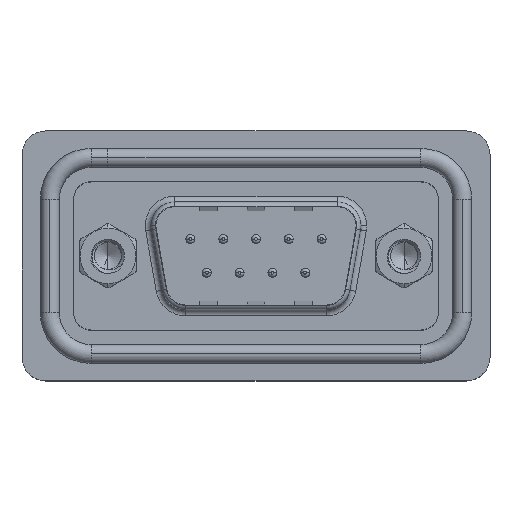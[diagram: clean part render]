
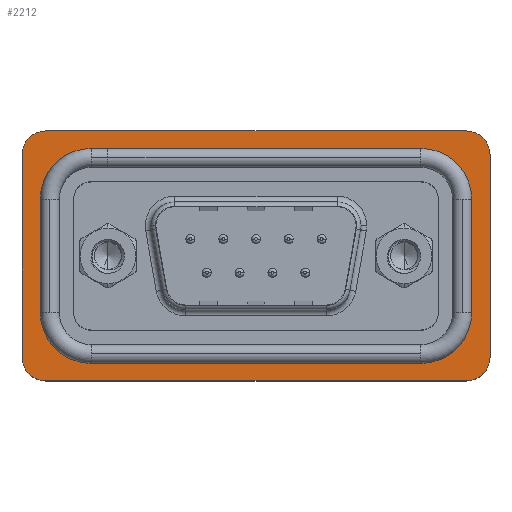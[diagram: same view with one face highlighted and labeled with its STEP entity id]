
A CAD part, top view. The second image highlights one B-rep face of the part: STEP entity #2212.
In plain terms, the highlighted planar face has unit normal (0, 0, 1).
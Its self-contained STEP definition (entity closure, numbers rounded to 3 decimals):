
#7 = DIRECTION ( 'NONE',  ( 1., 0., 0. ) ) ;
#293 = VERTEX_POINT ( 'NONE', #15740 ) ;
#303 = DIRECTION ( 'NONE',  ( 0., -1., 0. ) ) ;
#667 = LINE ( 'NONE', #5369, #3096 ) ;
#698 = CARTESIAN_POINT ( 'NONE',  ( 26.405, 9.075, 0.5 ) ) ;
#702 = CARTESIAN_POINT ( 'NONE',  ( -5.25, 10.55, 0.5 ) ) ;
#779 = VERTEX_POINT ( 'NONE', #1480 ) ;
#960 = CARTESIAN_POINT ( 'NONE',  ( -5.25, -8.55, 0.5 ) ) ;
#1004 = CARTESIAN_POINT ( 'NONE',  ( 26.405, -9.075, 0.5 ) ) ;
#1094 = VECTOR ( 'NONE', #3246, 1000. ) ;
#1358 = ORIENTED_EDGE ( 'NONE', *, *, #5745, .F. ) ;
#1480 = CARTESIAN_POINT ( 'NONE',  ( 30.705, -4.775, 0.5 ) ) ;
#1558 = CIRCLE ( 'NONE', #3838, 2. ) ;
#1612 = ORIENTED_EDGE ( 'NONE', *, *, #15712, .F. ) ;
#1641 = CARTESIAN_POINT ( 'NONE',  ( -1.405, 9.075, 0.5 ) ) ;
#1839 = LINE ( 'NONE', #8086, #11304 ) ;
#2130 = LINE ( 'NONE', #15849, #5525 ) ;
#2212 = ADVANCED_FACE ( 'NONE', ( #6549, #6759 ), #11276, .T. ) ;
#2410 = AXIS2_PLACEMENT_3D ( 'NONE', #3085, #6654, #7 ) ;
#2508 = VERTEX_POINT ( 'NONE', #20027 ) ;
#2511 = DIRECTION ( 'NONE',  ( -1., 0., 0. ) ) ;
#2998 = EDGE_CURVE ( 'NONE', #5143, #14491, #10978, .T. ) ;
#3085 = CARTESIAN_POINT ( 'NONE',  ( -1.405, -4.775, 0.5 ) ) ;
#3096 = VECTOR ( 'NONE', #2511, 1000. ) ;
#3149 = LINE ( 'NONE', #4671, #8349 ) ;
#3159 = ORIENTED_EDGE ( 'NONE', *, *, #10698, .T. ) ;
#3246 = DIRECTION ( 'NONE',  ( 0., 1., 0. ) ) ;
#3379 = DIRECTION ( 'NONE',  ( 1., 0., 0. ) ) ;
#3398 = VECTOR ( 'NONE', #16987, 1000. ) ;
#3555 = DIRECTION ( 'NONE',  ( 1., 0., 0. ) ) ;
#3666 = DIRECTION ( 'NONE',  ( 0., 0., 1. ) ) ;
#3838 = AXIS2_PLACEMENT_3D ( 'NONE', #17685, #3666, #9921 ) ;
#3862 = EDGE_CURVE ( 'NONE', #11667, #16319, #6385, .T. ) ;
#3866 = CIRCLE ( 'NONE', #14004, 2. ) ;
#3892 = CARTESIAN_POINT ( 'NONE',  ( 32.25, -8.55, 0.5 ) ) ;
#4145 = ORIENTED_EDGE ( 'NONE', *, *, #11080, .F. ) ;
#4476 = CIRCLE ( 'NONE', #15607, 2. ) ;
#4671 = CARTESIAN_POINT ( 'NONE',  ( 30.25, -10.55, 0.5 ) ) ;
#4672 = CARTESIAN_POINT ( 'NONE',  ( -1.405, 4.775, 0.5 ) ) ;
#5143 = VERTEX_POINT ( 'NONE', #17785 ) ;
#5189 = DIRECTION ( 'NONE',  ( 0., 0., 1. ) ) ;
#5277 = DIRECTION ( 'NONE',  ( 0., -1., 0. ) ) ;
#5358 = ORIENTED_EDGE ( 'NONE', *, *, #17830, .F. ) ;
#5361 = VERTEX_POINT ( 'NONE', #13994 ) ;
#5369 = CARTESIAN_POINT ( 'NONE',  ( 30.25, 10.55, 0.5 ) ) ;
#5525 = VECTOR ( 'NONE', #12693, 1000. ) ;
#5574 = EDGE_CURVE ( 'NONE', #16319, #2508, #9483, .T. ) ;
#5633 = VECTOR ( 'NONE', #5277, 1000. ) ;
#5745 = EDGE_CURVE ( 'NONE', #293, #19605, #14707, .T. ) ;
#5815 = VERTEX_POINT ( 'NONE', #11754 ) ;
#6047 = AXIS2_PLACEMENT_3D ( 'NONE', #16203, #12932, #17631 ) ;
#6385 = CIRCLE ( 'NONE', #17832, 2. ) ;
#6549 = FACE_BOUND ( 'NONE', #17944, .T. ) ;
#6555 = EDGE_CURVE ( 'NONE', #19605, #9737, #18405, .T. ) ;
#6643 = CARTESIAN_POINT ( 'NONE',  ( 30.25, 8.55, 0.5 ) ) ;
#6654 = DIRECTION ( 'NONE',  ( 0., 0., 1. ) ) ;
#6759 = FACE_OUTER_BOUND ( 'NONE', #15097, .T. ) ;
#6971 = CARTESIAN_POINT ( 'NONE',  ( 30.705, -4.775, 0.5 ) ) ;
#7002 = AXIS2_PLACEMENT_3D ( 'NONE', #6643, #9744, #3379 ) ;
#7195 = DIRECTION ( 'NONE',  ( 0., 0., 1. ) ) ;
#7319 = EDGE_CURVE ( 'NONE', #15814, #10655, #667, .T. ) ;
#7572 = LINE ( 'NONE', #15462, #3398 ) ;
#8086 = CARTESIAN_POINT ( 'NONE',  ( -7.25, -8.55, 0.5 ) ) ;
#8247 = CARTESIAN_POINT ( 'NONE',  ( 32.25, -8.55, 0.5 ) ) ;
#8293 = CARTESIAN_POINT ( 'NONE',  ( 30.25, -8.55, 0.5 ) ) ;
#8349 = VECTOR ( 'NONE', #12568, 1000. ) ;
#8527 = ORIENTED_EDGE ( 'NONE', *, *, #17581, .T. ) ;
#8582 = EDGE_CURVE ( 'NONE', #10655, #5815, #4476, .T. ) ;
#8651 = CARTESIAN_POINT ( 'NONE',  ( -5.705, 4.775, 0.5 ) ) ;
#8803 = CARTESIAN_POINT ( 'NONE',  ( -5.25, 8.55, 0.5 ) ) ;
#9399 = CIRCLE ( 'NONE', #13975, 4.3 ) ;
#9483 = LINE ( 'NONE', #8247, #1094 ) ;
#9565 = ORIENTED_EDGE ( 'NONE', *, *, #5574, .T. ) ;
#9657 = AXIS2_PLACEMENT_3D ( 'NONE', #15427, #15731, #20118 ) ;
#9737 = VERTEX_POINT ( 'NONE', #15664 ) ;
#9744 = DIRECTION ( 'NONE',  ( 0., 0., 1. ) ) ;
#9921 = DIRECTION ( 'NONE',  ( 1., 0., 0. ) ) ;
#10398 = ORIENTED_EDGE ( 'NONE', *, *, #2998, .F. ) ;
#10655 = VERTEX_POINT ( 'NONE', #702 ) ;
#10698 = EDGE_CURVE ( 'NONE', #2508, #15814, #1558, .T. ) ;
#10743 = DIRECTION ( 'NONE',  ( 0., 0., 1. ) ) ;
#10783 = VERTEX_POINT ( 'NONE', #1004 ) ;
#10978 = CIRCLE ( 'NONE', #6047, 4.3 ) ;
#11014 = CARTESIAN_POINT ( 'NONE',  ( -5.705, -4.775, 0.5 ) ) ;
#11080 = EDGE_CURVE ( 'NONE', #11955, #293, #9399, .T. ) ;
#11276 = PLANE ( 'NONE',  #7002 ) ;
#11304 = VECTOR ( 'NONE', #303, 1000. ) ;
#11609 = LINE ( 'NONE', #6971, #14509 ) ;
#11667 = VERTEX_POINT ( 'NONE', #12847 ) ;
#11754 = CARTESIAN_POINT ( 'NONE',  ( -7.25, 8.55, 0.5 ) ) ;
#11765 = EDGE_CURVE ( 'NONE', #17710, #5361, #3866, .T. ) ;
#11808 = ORIENTED_EDGE ( 'NONE', *, *, #11765, .T. ) ;
#11955 = VERTEX_POINT ( 'NONE', #1641 ) ;
#12568 = DIRECTION ( 'NONE',  ( 1., 0., 0. ) ) ;
#12669 = EDGE_CURVE ( 'NONE', #9737, #10783, #2130, .T. ) ;
#12693 = DIRECTION ( 'NONE',  ( 1., 0., 0. ) ) ;
#12847 = CARTESIAN_POINT ( 'NONE',  ( 30.25, -10.55, 0.5 ) ) ;
#12932 = DIRECTION ( 'NONE',  ( 0., 0., 1. ) ) ;
#13081 = ORIENTED_EDGE ( 'NONE', *, *, #7319, .T. ) ;
#13525 = DIRECTION ( 'NONE',  ( 0., 1., 0. ) ) ;
#13901 = CIRCLE ( 'NONE', #9657, 4.3 ) ;
#13975 = AXIS2_PLACEMENT_3D ( 'NONE', #4672, #5189, #3555 ) ;
#13994 = CARTESIAN_POINT ( 'NONE',  ( -5.25, -10.55, 0.5 ) ) ;
#14004 = AXIS2_PLACEMENT_3D ( 'NONE', #960, #7195, #16983 ) ;
#14094 = CARTESIAN_POINT ( 'NONE',  ( -7.25, -8.55, 0.5 ) ) ;
#14473 = ORIENTED_EDGE ( 'NONE', *, *, #12669, .F. ) ;
#14491 = VERTEX_POINT ( 'NONE', #698 ) ;
#14509 = VECTOR ( 'NONE', #13525, 1000. ) ;
#14707 = LINE ( 'NONE', #8651, #5633 ) ;
#14765 = CARTESIAN_POINT ( 'NONE',  ( 30.25, 10.55, 0.5 ) ) ;
#15097 = EDGE_LOOP ( 'NONE', ( #3159, #13081, #20128, #8527, #11808, #18176, #20076, #9565 ) ) ;
#15152 = ORIENTED_EDGE ( 'NONE', *, *, #6555, .F. ) ;
#15427 = CARTESIAN_POINT ( 'NONE',  ( 26.405, -4.775, 0.5 ) ) ;
#15462 = CARTESIAN_POINT ( 'NONE',  ( 26.405, 9.075, 0.5 ) ) ;
#15607 = AXIS2_PLACEMENT_3D ( 'NONE', #8803, #10743, #16972 ) ;
#15664 = CARTESIAN_POINT ( 'NONE',  ( -1.405, -9.075, 0.5 ) ) ;
#15712 = EDGE_CURVE ( 'NONE', #779, #5143, #11609, .T. ) ;
#15731 = DIRECTION ( 'NONE',  ( 0., 0., 1. ) ) ;
#15740 = CARTESIAN_POINT ( 'NONE',  ( -5.705, 4.775, 0.5 ) ) ;
#15814 = VERTEX_POINT ( 'NONE', #14765 ) ;
#15836 = EDGE_CURVE ( 'NONE', #14491, #11955, #7572, .T. ) ;
#15849 = CARTESIAN_POINT ( 'NONE',  ( -1.405, -9.075, 0.5 ) ) ;
#15873 = DIRECTION ( 'NONE',  ( 0., 0., 1. ) ) ;
#16203 = CARTESIAN_POINT ( 'NONE',  ( 26.405, 4.775, 0.5 ) ) ;
#16319 = VERTEX_POINT ( 'NONE', #3892 ) ;
#16972 = DIRECTION ( 'NONE',  ( 1., 0., 0. ) ) ;
#16983 = DIRECTION ( 'NONE',  ( -1., 0., 0. ) ) ;
#16987 = DIRECTION ( 'NONE',  ( -1., 0., 0. ) ) ;
#17581 = EDGE_CURVE ( 'NONE', #5815, #17710, #1839, .T. ) ;
#17631 = DIRECTION ( 'NONE',  ( 1., 0., 0. ) ) ;
#17685 = CARTESIAN_POINT ( 'NONE',  ( 30.25, 8.55, 0.5 ) ) ;
#17710 = VERTEX_POINT ( 'NONE', #14094 ) ;
#17785 = CARTESIAN_POINT ( 'NONE',  ( 30.705, 4.775, 0.5 ) ) ;
#17830 = EDGE_CURVE ( 'NONE', #10783, #779, #13901, .T. ) ;
#17832 = AXIS2_PLACEMENT_3D ( 'NONE', #8293, #15873, #19038 ) ;
#17944 = EDGE_LOOP ( 'NONE', ( #10398, #1612, #5358, #14473, #15152, #1358, #4145, #18035 ) ) ;
#18035 = ORIENTED_EDGE ( 'NONE', *, *, #15836, .F. ) ;
#18176 = ORIENTED_EDGE ( 'NONE', *, *, #19070, .T. ) ;
#18405 = CIRCLE ( 'NONE', #2410, 4.3 ) ;
#19038 = DIRECTION ( 'NONE',  ( 1., 0., 0. ) ) ;
#19070 = EDGE_CURVE ( 'NONE', #5361, #11667, #3149, .T. ) ;
#19605 = VERTEX_POINT ( 'NONE', #11014 ) ;
#20027 = CARTESIAN_POINT ( 'NONE',  ( 32.25, 8.55, 0.5 ) ) ;
#20076 = ORIENTED_EDGE ( 'NONE', *, *, #3862, .T. ) ;
#20118 = DIRECTION ( 'NONE',  ( 1., 0., 0. ) ) ;
#20128 = ORIENTED_EDGE ( 'NONE', *, *, #8582, .T. ) ;
